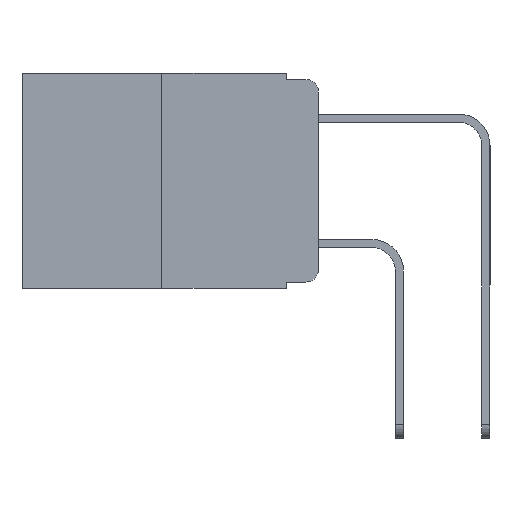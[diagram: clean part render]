
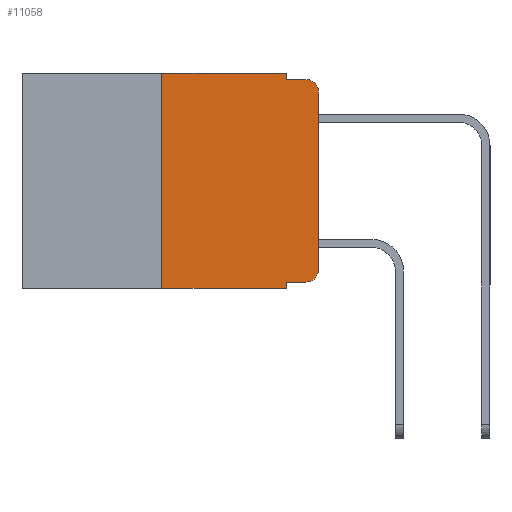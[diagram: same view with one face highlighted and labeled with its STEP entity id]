
A CAD part, left-side view. The second image highlights one B-rep face of the part: STEP entity #11058.
In plain terms, the highlighted planar face has unit normal (-1, 0, 0).
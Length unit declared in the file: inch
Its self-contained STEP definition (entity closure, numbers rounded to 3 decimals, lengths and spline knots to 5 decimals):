
#24 = CARTESIAN_POINT ( 'NONE',  ( 0., 0.051, -0.333 ) ) ;
#339 = VECTOR ( 'NONE', #8316, 39.37008 ) ;
#495 = AXIS2_PLACEMENT_3D ( 'NONE', #1431, #1444, #1491 ) ;
#557 = ORIENTED_EDGE ( 'NONE', *, *, #9607, .T. ) ;
#584 = PLANE ( 'NONE',  #2927 ) ;
#733 = CARTESIAN_POINT ( 'NONE',  ( 0., 0., -0.03 ) ) ;
#927 = ORIENTED_EDGE ( 'NONE', *, *, #9412, .F. ) ;
#1002 = VECTOR ( 'NONE', #8574, 39.37008 ) ;
#1104 = CARTESIAN_POINT ( 'NONE',  ( 0., 0., -0.313 ) ) ;
#1186 = DIRECTION ( 'NONE',  ( 0., -1., 0. ) ) ;
#1431 = CARTESIAN_POINT ( 'NONE',  ( 0., 0.02, -0.03 ) ) ;
#1444 = DIRECTION ( 'NONE',  ( -1., 0., 0. ) ) ;
#1457 = CARTESIAN_POINT ( 'NONE',  ( 0., 0.02, -0.313 ) ) ;
#1491 = DIRECTION ( 'NONE',  ( 0., 0., -1. ) ) ;
#1841 = VERTEX_POINT ( 'NONE', #2039 ) ;
#2039 = CARTESIAN_POINT ( 'NONE',  ( 0., 0.02, -0.01 ) ) ;
#2170 = VERTEX_POINT ( 'NONE', #6820 ) ;
#2234 = VERTEX_POINT ( 'NONE', #11591 ) ;
#2517 = VECTOR ( 'NONE', #4404, 39.37008 ) ;
#2539 = DIRECTION ( 'NONE',  ( 0., 0., -1. ) ) ;
#2658 = EDGE_CURVE ( 'NONE', #13663, #2170, #5451, .T. ) ;
#2771 = ORIENTED_EDGE ( 'NONE', *, *, #5505, .T. ) ;
#2927 = AXIS2_PLACEMENT_3D ( 'NONE', #3908, #11380, #5025 ) ;
#3120 = FACE_OUTER_BOUND ( 'NONE', #10170, .T. ) ;
#3278 = LINE ( 'NONE', #8314, #339 ) ;
#3338 = VECTOR ( 'NONE', #9778, 39.37008 ) ;
#3560 = LINE ( 'NONE', #7495, #1002 ) ;
#3908 = CARTESIAN_POINT ( 'NONE',  ( 0., 0.473, 0. ) ) ;
#3945 = CARTESIAN_POINT ( 'NONE',  ( 0., 0.25, -0.343 ) ) ;
#4005 = DIRECTION ( 'NONE',  ( 0., 0., 1. ) ) ;
#4041 = LINE ( 'NONE', #13876, #3338 ) ;
#4051 = AXIS2_PLACEMENT_3D ( 'NONE', #1457, #9012, #2539 ) ;
#4122 = CARTESIAN_POINT ( 'NONE',  ( 0., 0.25, 0. ) ) ;
#4404 = DIRECTION ( 'NONE',  ( 0., 0., -1. ) ) ;
#4450 = CARTESIAN_POINT ( 'NONE',  ( 0., 0.051, -0.343 ) ) ;
#4887 = EDGE_CURVE ( 'NONE', #6108, #1841, #4041, .T. ) ;
#4926 = VERTEX_POINT ( 'NONE', #733 ) ;
#5025 = DIRECTION ( 'NONE',  ( 0., 0., -1. ) ) ;
#5233 = EDGE_CURVE ( 'NONE', #8304, #6243, #7557, .T. ) ;
#5421 = CARTESIAN_POINT ( 'NONE',  ( 0., 0.051, 0. ) ) ;
#5451 = LINE ( 'NONE', #7947, #6941 ) ;
#5505 = EDGE_CURVE ( 'NONE', #4926, #1841, #7049, .T. ) ;
#5819 = LINE ( 'NONE', #8286, #8350 ) ;
#5929 = CIRCLE ( 'NONE', #4051, 0.02 ) ;
#6108 = VERTEX_POINT ( 'NONE', #12921 ) ;
#6220 = EDGE_CURVE ( 'NONE', #2234, #6108, #12658, .T. ) ;
#6243 = VERTEX_POINT ( 'NONE', #4450 ) ;
#6559 = ORIENTED_EDGE ( 'NONE', *, *, #5233, .T. ) ;
#6820 = CARTESIAN_POINT ( 'NONE',  ( 0., 0.02, -0.333 ) ) ;
#6941 = VECTOR ( 'NONE', #12715, 39.37008 ) ;
#6947 = EDGE_CURVE ( 'NONE', #10065, #4926, #3278, .T. ) ;
#7027 = VECTOR ( 'NONE', #9263, 39.37008 ) ;
#7049 = CIRCLE ( 'NONE', #495, 0.02 ) ;
#7371 = ORIENTED_EDGE ( 'NONE', *, *, #6947, .T. ) ;
#7383 = ORIENTED_EDGE ( 'NONE', *, *, #2658, .T. ) ;
#7495 = CARTESIAN_POINT ( 'NONE',  ( 0., 0.473, 0. ) ) ;
#7557 = LINE ( 'NONE', #13913, #12854 ) ;
#7947 = CARTESIAN_POINT ( 'NONE',  ( 0., 0.051, -0.333 ) ) ;
#8286 = CARTESIAN_POINT ( 'NONE',  ( 0., 0.25, 0. ) ) ;
#8299 = LINE ( 'NONE', #8617, #2517 ) ;
#8304 = VERTEX_POINT ( 'NONE', #3945 ) ;
#8314 = CARTESIAN_POINT ( 'NONE',  ( 0., 0., 0. ) ) ;
#8316 = DIRECTION ( 'NONE',  ( 0., 0., 1. ) ) ;
#8350 = VECTOR ( 'NONE', #4005, 39.37008 ) ;
#8574 = DIRECTION ( 'NONE',  ( 0., -1., 0. ) ) ;
#8617 = CARTESIAN_POINT ( 'NONE',  ( 0., 0.051, 0. ) ) ;
#8726 = ORIENTED_EDGE ( 'NONE', *, *, #9355, .F. ) ;
#9012 = DIRECTION ( 'NONE',  ( -1., 0., 0. ) ) ;
#9263 = DIRECTION ( 'NONE',  ( 0., 0., -1. ) ) ;
#9355 = EDGE_CURVE ( 'NONE', #10535, #2234, #3560, .T. ) ;
#9412 = EDGE_CURVE ( 'NONE', #13663, #6243, #8299, .T. ) ;
#9607 = EDGE_CURVE ( 'NONE', #2170, #10065, #5929, .T. ) ;
#9712 = ORIENTED_EDGE ( 'NONE', *, *, #4887, .F. ) ;
#9778 = DIRECTION ( 'NONE',  ( 0., -1., 0. ) ) ;
#10065 = VERTEX_POINT ( 'NONE', #1104 ) ;
#10170 = EDGE_LOOP ( 'NONE', ( #7371, #2771, #9712, #13689, #8726, #11869, #6559, #927, #7383, #557 ) ) ;
#10535 = VERTEX_POINT ( 'NONE', #4122 ) ;
#11058 = ADVANCED_FACE ( 'NONE', ( #3120 ), #584, .F. ) ;
#11380 = DIRECTION ( 'NONE',  ( 1., 0., 0. ) ) ;
#11591 = CARTESIAN_POINT ( 'NONE',  ( 0., 0.051, 0. ) ) ;
#11677 = EDGE_CURVE ( 'NONE', #8304, #10535, #5819, .T. ) ;
#11869 = ORIENTED_EDGE ( 'NONE', *, *, #11677, .F. ) ;
#12658 = LINE ( 'NONE', #5421, #7027 ) ;
#12715 = DIRECTION ( 'NONE',  ( 0., -1., 0. ) ) ;
#12854 = VECTOR ( 'NONE', #1186, 39.37008 ) ;
#12921 = CARTESIAN_POINT ( 'NONE',  ( 0., 0.051, -0.01 ) ) ;
#13663 = VERTEX_POINT ( 'NONE', #24 ) ;
#13689 = ORIENTED_EDGE ( 'NONE', *, *, #6220, .F. ) ;
#13876 = CARTESIAN_POINT ( 'NONE',  ( 0., 0.051, -0.01 ) ) ;
#13913 = CARTESIAN_POINT ( 'NONE',  ( 0., 0.473, -0.343 ) ) ;
